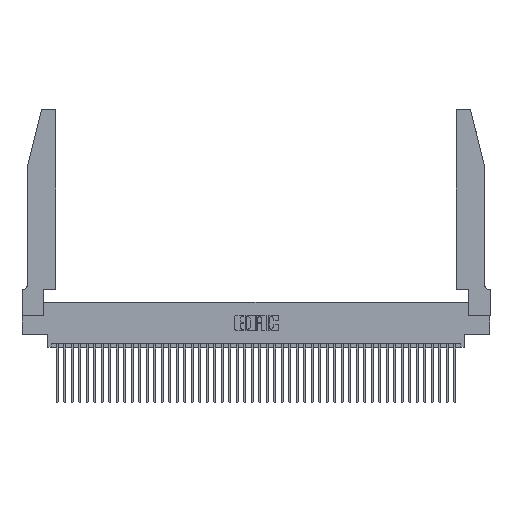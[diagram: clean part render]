
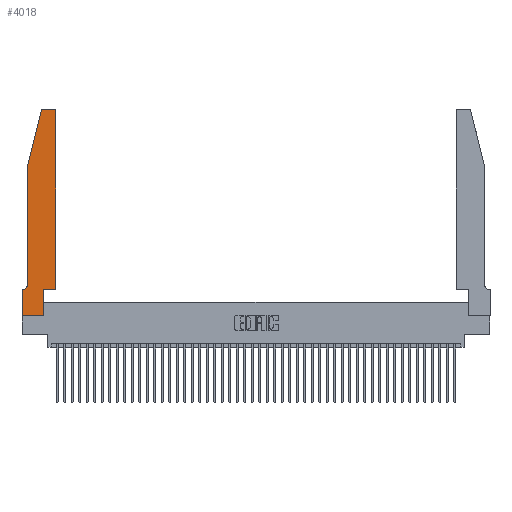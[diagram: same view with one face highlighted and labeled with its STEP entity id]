
A CAD part, top view. The second image highlights one B-rep face of the part: STEP entity #4018.
In plain terms, the highlighted planar face has unit normal (0, 0, 1).
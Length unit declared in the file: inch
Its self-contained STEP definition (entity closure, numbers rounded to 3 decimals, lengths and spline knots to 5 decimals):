
#460 = DIRECTION ( 'NONE',  ( 0., 0., 1. ) ) ;
#2231 = LINE ( 'NONE', #11377, #8258 ) ;
#2379 = VECTOR ( 'NONE', #16370, 39.37008 ) ;
#3554 = CARTESIAN_POINT ( 'NONE',  ( 0., 0.35, 0.37 ) ) ;
#3704 = AXIS2_PLACEMENT_3D ( 'NONE', #32924, #40006, #40160 ) ;
#3711 = CARTESIAN_POINT ( 'NONE',  ( 0.284, 2.72, 0.37 ) ) ;
#4018 = ADVANCED_FACE ( 'NONE', ( #6322 ), #14086, .T. ) ;
#4259 = ORIENTED_EDGE ( 'NONE', *, *, #24728, .T. ) ;
#4924 = CIRCLE ( 'NONE', #40969, 0.03 ) ;
#5295 = VERTEX_POINT ( 'NONE', #14886 ) ;
#5327 = VERTEX_POINT ( 'NONE', #42897 ) ;
#5720 = VERTEX_POINT ( 'NONE', #27610 ) ;
#6322 = FACE_OUTER_BOUND ( 'NONE', #30172, .T. ) ;
#6719 = CARTESIAN_POINT ( 'NONE',  ( 0.25487, 2.72718, 0.37 ) ) ;
#7101 = DIRECTION ( 'NONE',  ( 1., 0., 0. ) ) ;
#7674 = LINE ( 'NONE', #24684, #12678 ) ;
#8042 = LINE ( 'NONE', #36007, #37852 ) ;
#8107 = CARTESIAN_POINT ( 'NONE',  ( 0., 0., 0.37 ) ) ;
#8258 = VECTOR ( 'NONE', #42944, 39.37008 ) ;
#8864 = ORIENTED_EDGE ( 'NONE', *, *, #15849, .T. ) ;
#9912 = CARTESIAN_POINT ( 'NONE',  ( 0., 0., 0.37 ) ) ;
#10076 = CIRCLE ( 'NONE', #3704, 0.03 ) ;
#10588 = ORIENTED_EDGE ( 'NONE', *, *, #45436, .T. ) ;
#10611 = CARTESIAN_POINT ( 'NONE',  ( 0.4505, 0.35, 0.37 ) ) ;
#10665 = ORIENTED_EDGE ( 'NONE', *, *, #36781, .T. ) ;
#10691 = DIRECTION ( 'NONE',  ( -1., 0., 0. ) ) ;
#11377 = CARTESIAN_POINT ( 'NONE',  ( 0., 0., 0.37 ) ) ;
#12436 = LINE ( 'NONE', #35177, #32285 ) ;
#12678 = VECTOR ( 'NONE', #35473, 39.37008 ) ;
#14022 = VECTOR ( 'NONE', #30808, 39.37008 ) ;
#14025 = VERTEX_POINT ( 'NONE', #10611 ) ;
#14086 = PLANE ( 'NONE',  #15426 ) ;
#14318 = EDGE_CURVE ( 'NONE', #38652, #41690, #44266, .T. ) ;
#14865 = LINE ( 'NONE', #40433, #40222 ) ;
#14886 = CARTESIAN_POINT ( 'NONE',  ( 0.4205, 2.75, 0.37 ) ) ;
#15426 = AXIS2_PLACEMENT_3D ( 'NONE', #3554, #460, #7101 ) ;
#15849 = EDGE_CURVE ( 'NONE', #36846, #14025, #7674, .T. ) ;
#16314 = VECTOR ( 'NONE', #17596, 39.37008 ) ;
#16370 = DIRECTION ( 'NONE',  ( 0., 1., 0. ) ) ;
#17596 = DIRECTION ( 'NONE',  ( 0., 1., 0. ) ) ;
#17794 = VERTEX_POINT ( 'NONE', #31918 ) ;
#19950 = VERTEX_POINT ( 'NONE', #24685 ) ;
#20369 = CARTESIAN_POINT ( 'NONE',  ( 0.2865, 0.35, 0.37 ) ) ;
#21389 = EDGE_CURVE ( 'NONE', #5327, #21531, #8042, .T. ) ;
#21531 = VERTEX_POINT ( 'NONE', #40137 ) ;
#22718 = EDGE_CURVE ( 'NONE', #24484, #19950, #45435, .T. ) ;
#23107 = EDGE_CURVE ( 'NONE', #17794, #5295, #10076, .T. ) ;
#23447 = ORIENTED_EDGE ( 'NONE', *, *, #34591, .T. ) ;
#24484 = VERTEX_POINT ( 'NONE', #44523 ) ;
#24684 = CARTESIAN_POINT ( 'NONE',  ( 0.4505, 0.35, 0.37 ) ) ;
#24685 = CARTESIAN_POINT ( 'NONE',  ( 0., 0.35, 0.37 ) ) ;
#24728 = EDGE_CURVE ( 'NONE', #19950, #38652, #2231, .T. ) ;
#25343 = DIRECTION ( 'NONE',  ( 0., -1., 0. ) ) ;
#25554 = LINE ( 'NONE', #33023, #2379 ) ;
#25843 = DIRECTION ( 'NONE',  ( 1., 0., 0. ) ) ;
#26083 = DIRECTION ( 'NONE',  ( -0.239, -0.971, 0. ) ) ;
#26239 = CIRCLE ( 'NONE', #26683, 0.07 ) ;
#26683 = AXIS2_PLACEMENT_3D ( 'NONE', #28263, #42440, #10691 ) ;
#27610 = CARTESIAN_POINT ( 'NONE',  ( 0.284, 2.75, 0.37 ) ) ;
#27688 = CARTESIAN_POINT ( 'NONE',  ( 0.2865, 0., 0.37 ) ) ;
#27696 = CARTESIAN_POINT ( 'NONE',  ( 0.0755, 0.35, 0.37 ) ) ;
#28263 = CARTESIAN_POINT ( 'NONE',  ( 0.0055, 0.42, 0.37 ) ) ;
#28555 = DIRECTION ( 'NONE',  ( 1., 0., 0. ) ) ;
#28857 = ORIENTED_EDGE ( 'NONE', *, *, #21389, .T. ) ;
#29143 = ORIENTED_EDGE ( 'NONE', *, *, #31867, .T. ) ;
#30172 = EDGE_LOOP ( 'NONE', ( #36702, #10588, #23447, #28857, #29143, #36092, #4259, #38514, #10665, #8864, #34716, #36596 ) ) ;
#30640 = LINE ( 'NONE', #20369, #16314 ) ;
#30808 = DIRECTION ( 'NONE',  ( -1., 0., 0. ) ) ;
#31867 = EDGE_CURVE ( 'NONE', #21531, #24484, #26239, .T. ) ;
#31918 = CARTESIAN_POINT ( 'NONE',  ( 0.4505, 2.72, 0.37 ) ) ;
#32285 = VECTOR ( 'NONE', #38264, 39.37008 ) ;
#32924 = CARTESIAN_POINT ( 'NONE',  ( 0.4205, 2.72, 0.37 ) ) ;
#33023 = CARTESIAN_POINT ( 'NONE',  ( 0.4505, 0.35, 0.37 ) ) ;
#33069 = VERTEX_POINT ( 'NONE', #6719 ) ;
#34591 = EDGE_CURVE ( 'NONE', #33069, #5327, #14865, .T. ) ;
#34716 = ORIENTED_EDGE ( 'NONE', *, *, #40860, .T. ) ;
#35177 = CARTESIAN_POINT ( 'NONE',  ( 0.2605, 2.75, 0.37 ) ) ;
#35473 = DIRECTION ( 'NONE',  ( 1., 0., 0. ) ) ;
#35486 = DIRECTION ( 'NONE',  ( 0., 0., 1. ) ) ;
#36007 = CARTESIAN_POINT ( 'NONE',  ( 0.0755, 2., 0.37 ) ) ;
#36092 = ORIENTED_EDGE ( 'NONE', *, *, #22718, .T. ) ;
#36596 = ORIENTED_EDGE ( 'NONE', *, *, #23107, .T. ) ;
#36702 = ORIENTED_EDGE ( 'NONE', *, *, #36852, .T. ) ;
#36781 = EDGE_CURVE ( 'NONE', #41690, #36846, #30640, .T. ) ;
#36846 = VERTEX_POINT ( 'NONE', #45493 ) ;
#36852 = EDGE_CURVE ( 'NONE', #5295, #5720, #12436, .T. ) ;
#37852 = VECTOR ( 'NONE', #25343, 39.37008 ) ;
#38264 = DIRECTION ( 'NONE',  ( -1., 0., 0. ) ) ;
#38514 = ORIENTED_EDGE ( 'NONE', *, *, #14318, .T. ) ;
#38652 = VERTEX_POINT ( 'NONE', #9912 ) ;
#40006 = DIRECTION ( 'NONE',  ( 0., 0., 1. ) ) ;
#40137 = CARTESIAN_POINT ( 'NONE',  ( 0.0755, 0.42, 0.37 ) ) ;
#40160 = DIRECTION ( 'NONE',  ( 1., 0., 0. ) ) ;
#40222 = VECTOR ( 'NONE', #26083, 39.37008 ) ;
#40433 = CARTESIAN_POINT ( 'NONE',  ( 0.0755, 2., 0.37 ) ) ;
#40860 = EDGE_CURVE ( 'NONE', #14025, #17794, #25554, .T. ) ;
#40969 = AXIS2_PLACEMENT_3D ( 'NONE', #3711, #35486, #28555 ) ;
#41690 = VERTEX_POINT ( 'NONE', #27688 ) ;
#42440 = DIRECTION ( 'NONE',  ( 0., 0., -1. ) ) ;
#42897 = CARTESIAN_POINT ( 'NONE',  ( 0.0755, 2., 0.37 ) ) ;
#42944 = DIRECTION ( 'NONE',  ( 0., -1., 0. ) ) ;
#44266 = LINE ( 'NONE', #8107, #44780 ) ;
#44523 = CARTESIAN_POINT ( 'NONE',  ( 0.0055, 0.35, 0.37 ) ) ;
#44780 = VECTOR ( 'NONE', #25843, 39.37008 ) ;
#45435 = LINE ( 'NONE', #27696, #14022 ) ;
#45436 = EDGE_CURVE ( 'NONE', #5720, #33069, #4924, .T. ) ;
#45493 = CARTESIAN_POINT ( 'NONE',  ( 0.2865, 0.35, 0.37 ) ) ;
